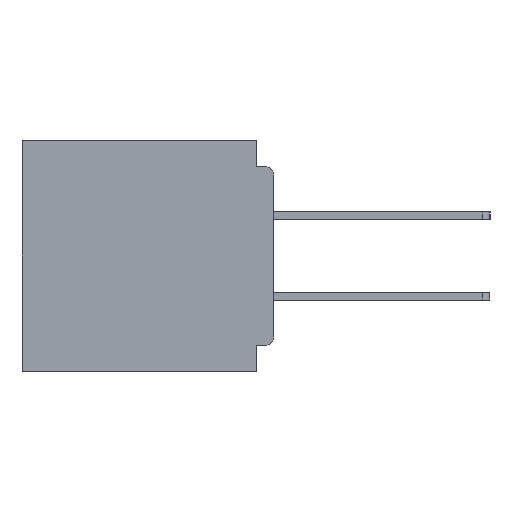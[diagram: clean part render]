
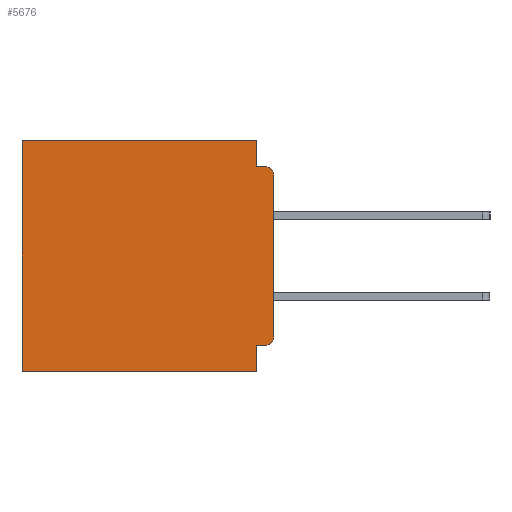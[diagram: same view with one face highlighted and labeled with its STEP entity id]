
A CAD part, left-side view. The second image highlights one B-rep face of the part: STEP entity #5676.
In plain terms, the highlighted planar face has unit normal (-1, 0, 0).
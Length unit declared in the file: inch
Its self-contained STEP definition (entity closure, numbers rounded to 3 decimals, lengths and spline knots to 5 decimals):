
#279 = LINE ( 'NONE', #45660, #50884 ) ;
#728 = DIRECTION ( 'NONE',  ( 0., 0., -1. ) ) ;
#868 = ORIENTED_EDGE ( 'NONE', *, *, #55656, .T. ) ;
#1183 = PLANE ( 'NONE',  #26390 ) ;
#2230 = CARTESIAN_POINT ( 'NONE',  ( 0.3, 0.031, -0.4 ) ) ;
#4647 = AXIS2_PLACEMENT_3D ( 'NONE', #59413, #30127, #728 ) ;
#5278 = CARTESIAN_POINT ( 'NONE',  ( 0.3, 0.437, 0. ) ) ;
#5676 = ADVANCED_FACE ( 'NONE', ( #16980 ), #1183, .F. ) ;
#6122 = DIRECTION ( 'NONE',  ( 0., 0., -1. ) ) ;
#8570 = ORIENTED_EDGE ( 'NONE', *, *, #37457, .T. ) ;
#10607 = CARTESIAN_POINT ( 'NONE',  ( 0.3, 0.437, -0.4 ) ) ;
#12461 = LINE ( 'NONE', #47359, #14009 ) ;
#12486 = CARTESIAN_POINT ( 'NONE',  ( 0.3, 0.031, 0. ) ) ;
#13143 = CARTESIAN_POINT ( 'NONE',  ( 0.3, 0.437, -0.4 ) ) ;
#13721 = VECTOR ( 'NONE', #25773, 39.37008 ) ;
#14009 = VECTOR ( 'NONE', #18039, 39.37008 ) ;
#16936 = EDGE_CURVE ( 'NONE', #45849, #57076, #53869, .T. ) ;
#16980 = FACE_OUTER_BOUND ( 'NONE', #18334, .T. ) ;
#18039 = DIRECTION ( 'NONE',  ( 0., 1., 0. ) ) ;
#18334 = EDGE_LOOP ( 'NONE', ( #45334, #868, #53004, #33127, #8570, #47660, #53800, #20912, #59937, #22427 ) ) ;
#18705 = DIRECTION ( 'NONE',  ( -1., 0., 0. ) ) ;
#19072 = CARTESIAN_POINT ( 'NONE',  ( 0.3, 0.031, -0.045 ) ) ;
#19268 = DIRECTION ( 'NONE',  ( 0., 1., 0. ) ) ;
#20912 = ORIENTED_EDGE ( 'NONE', *, *, #24548, .F. ) ;
#22427 = ORIENTED_EDGE ( 'NONE', *, *, #31907, .T. ) ;
#22495 = VECTOR ( 'NONE', #45069, 39.37008 ) ;
#22729 = VERTEX_POINT ( 'NONE', #60583 ) ;
#24004 = LINE ( 'NONE', #12486, #35523 ) ;
#24120 = LINE ( 'NONE', #29084, #38727 ) ;
#24548 = EDGE_CURVE ( 'NONE', #39541, #45849, #279, .T. ) ;
#25195 = VECTOR ( 'NONE', #47391, 39.37008 ) ;
#25567 = CARTESIAN_POINT ( 'NONE',  ( 0.3, 0., -0.4 ) ) ;
#25635 = CARTESIAN_POINT ( 'NONE',  ( 0.3, 0., -0.4 ) ) ;
#25773 = DIRECTION ( 'NONE',  ( 0., -1., 0. ) ) ;
#26058 = CARTESIAN_POINT ( 'NONE',  ( 0.3, 0.031, -0.355 ) ) ;
#26163 = DIRECTION ( 'NONE',  ( 0., 0., -1. ) ) ;
#26390 = AXIS2_PLACEMENT_3D ( 'NONE', #25635, #35513, #6122 ) ;
#27986 = VERTEX_POINT ( 'NONE', #54771 ) ;
#28646 = EDGE_CURVE ( 'NONE', #43195, #57076, #35183, .T. ) ;
#29084 = CARTESIAN_POINT ( 'NONE',  ( 0.3, 0., 0. ) ) ;
#30127 = DIRECTION ( 'NONE',  ( -1., 0., 0. ) ) ;
#31907 = EDGE_CURVE ( 'NONE', #22729, #37692, #61645, .T. ) ;
#32194 = AXIS2_PLACEMENT_3D ( 'NONE', #48016, #18705, #52931 ) ;
#32440 = LINE ( 'NONE', #25567, #22495 ) ;
#32658 = VERTEX_POINT ( 'NONE', #45034 ) ;
#33127 = ORIENTED_EDGE ( 'NONE', *, *, #38390, .F. ) ;
#35183 = LINE ( 'NONE', #13143, #25195 ) ;
#35513 = DIRECTION ( 'NONE',  ( 1., 0., 0. ) ) ;
#35523 = VECTOR ( 'NONE', #56585, 39.37008 ) ;
#35727 = VERTEX_POINT ( 'NONE', #19072 ) ;
#37457 = EDGE_CURVE ( 'NONE', #27986, #43195, #24120, .T. ) ;
#37608 = CARTESIAN_POINT ( 'NONE',  ( 0.3, 0.015, -0.045 ) ) ;
#37692 = VERTEX_POINT ( 'NONE', #60283 ) ;
#38390 = EDGE_CURVE ( 'NONE', #27986, #35727, #24004, .T. ) ;
#38727 = VECTOR ( 'NONE', #19268, 39.37008 ) ;
#39541 = VERTEX_POINT ( 'NONE', #26058 ) ;
#39551 = CIRCLE ( 'NONE', #32194, 0.015 ) ;
#39821 = LINE ( 'NONE', #55081, #13721 ) ;
#43195 = VERTEX_POINT ( 'NONE', #5278 ) ;
#43953 = EDGE_CURVE ( 'NONE', #32658, #37692, #32440, .T. ) ;
#44251 = EDGE_CURVE ( 'NONE', #22729, #39541, #12461, .T. ) ;
#45034 = CARTESIAN_POINT ( 'NONE',  ( 0.3, 0., -0.06 ) ) ;
#45069 = DIRECTION ( 'NONE',  ( 0., 0., -1. ) ) ;
#45334 = ORIENTED_EDGE ( 'NONE', *, *, #43953, .F. ) ;
#45660 = CARTESIAN_POINT ( 'NONE',  ( 0.3, 0.031, -0.4 ) ) ;
#45849 = VERTEX_POINT ( 'NONE', #2230 ) ;
#46291 = EDGE_CURVE ( 'NONE', #35727, #53598, #39821, .T. ) ;
#47359 = CARTESIAN_POINT ( 'NONE',  ( 0.3, 0., -0.355 ) ) ;
#47391 = DIRECTION ( 'NONE',  ( 0., 0., -1. ) ) ;
#47660 = ORIENTED_EDGE ( 'NONE', *, *, #28646, .T. ) ;
#48016 = CARTESIAN_POINT ( 'NONE',  ( 0.3, 0.015, -0.06 ) ) ;
#50884 = VECTOR ( 'NONE', #26163, 39.37008 ) ;
#52319 = VECTOR ( 'NONE', #59955, 39.37008 ) ;
#52931 = DIRECTION ( 'NONE',  ( 0., 0., -1. ) ) ;
#53004 = ORIENTED_EDGE ( 'NONE', *, *, #46291, .F. ) ;
#53598 = VERTEX_POINT ( 'NONE', #37608 ) ;
#53800 = ORIENTED_EDGE ( 'NONE', *, *, #16936, .F. ) ;
#53869 = LINE ( 'NONE', #55047, #52319 ) ;
#54771 = CARTESIAN_POINT ( 'NONE',  ( 0.3, 0.031, 0. ) ) ;
#55047 = CARTESIAN_POINT ( 'NONE',  ( 0.3, 0., -0.4 ) ) ;
#55081 = CARTESIAN_POINT ( 'NONE',  ( 0.3, 0., -0.045 ) ) ;
#55656 = EDGE_CURVE ( 'NONE', #32658, #53598, #39551, .T. ) ;
#56585 = DIRECTION ( 'NONE',  ( 0., 0., -1. ) ) ;
#57076 = VERTEX_POINT ( 'NONE', #10607 ) ;
#59413 = CARTESIAN_POINT ( 'NONE',  ( 0.3, 0.015, -0.34 ) ) ;
#59937 = ORIENTED_EDGE ( 'NONE', *, *, #44251, .F. ) ;
#59955 = DIRECTION ( 'NONE',  ( 0., 1., 0. ) ) ;
#60283 = CARTESIAN_POINT ( 'NONE',  ( 0.3, 0., -0.34 ) ) ;
#60583 = CARTESIAN_POINT ( 'NONE',  ( 0.3, 0.015, -0.355 ) ) ;
#61645 = CIRCLE ( 'NONE', #4647, 0.015 ) ;
